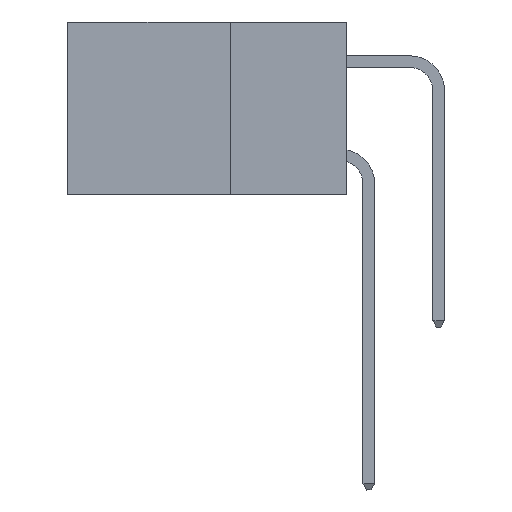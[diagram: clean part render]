
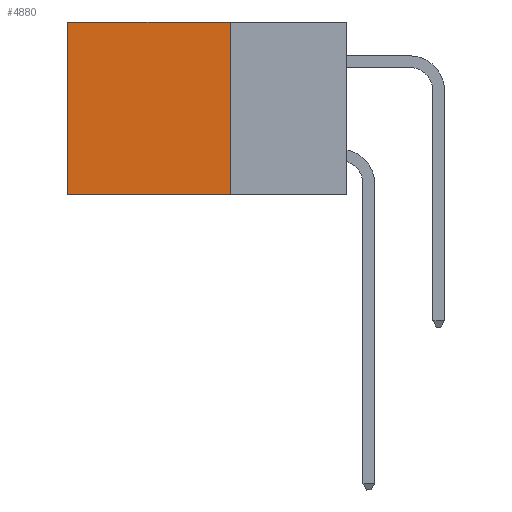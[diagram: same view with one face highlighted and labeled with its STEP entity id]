
A CAD part, left-side view. The second image highlights one B-rep face of the part: STEP entity #4880.
In plain terms, the highlighted planar face has unit normal (-1, 0, 0).
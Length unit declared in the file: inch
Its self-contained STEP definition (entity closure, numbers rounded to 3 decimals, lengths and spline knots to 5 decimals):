
#574 = CARTESIAN_POINT ( 'NONE',  ( 0.2875, 0.25, 0. ) ) ;
#4880 = ADVANCED_FACE ( 'NONE', ( #31165 ), #34774, .F. ) ;
#5216 = EDGE_LOOP ( 'NONE', ( #14999, #32293, #36524, #15111 ) ) ;
#5328 = DIRECTION ( 'NONE',  ( 0., 1., 0. ) ) ;
#6988 = DIRECTION ( 'NONE',  ( 0., 1., 0. ) ) ;
#8904 = VERTEX_POINT ( 'NONE', #18825 ) ;
#9302 = EDGE_CURVE ( 'NONE', #16765, #35006, #14857, .T. ) ;
#9684 = CARTESIAN_POINT ( 'NONE',  ( 0.2875, 0.25, 0. ) ) ;
#10990 = VECTOR ( 'NONE', #6988, 39.37008 ) ;
#11474 = DIRECTION ( 'NONE',  ( 1., 0., 0. ) ) ;
#12344 = EDGE_CURVE ( 'NONE', #27706, #8904, #24925, .T. ) ;
#14065 = LINE ( 'NONE', #31972, #17179 ) ;
#14857 = LINE ( 'NONE', #25021, #18879 ) ;
#14999 = ORIENTED_EDGE ( 'NONE', *, *, #33386, .T. ) ;
#15111 = ORIENTED_EDGE ( 'NONE', *, *, #12344, .T. ) ;
#16765 = VERTEX_POINT ( 'NONE', #18078 ) ;
#17179 = VECTOR ( 'NONE', #25967, 39.37008 ) ;
#18078 = CARTESIAN_POINT ( 'NONE',  ( 0.2875, 0.25, -0.37 ) ) ;
#18412 = CARTESIAN_POINT ( 'NONE',  ( 0.2875, 0.25, 0. ) ) ;
#18825 = CARTESIAN_POINT ( 'NONE',  ( 0.2875, 0.6, 0. ) ) ;
#18879 = VECTOR ( 'NONE', #5328, 39.37008 ) ;
#19658 = CARTESIAN_POINT ( 'NONE',  ( 0.2875, 0.6, -0.37 ) ) ;
#20330 = AXIS2_PLACEMENT_3D ( 'NONE', #574, #11474, #23914 ) ;
#23914 = DIRECTION ( 'NONE',  ( 0., 0., -1. ) ) ;
#24255 = DIRECTION ( 'NONE',  ( 0., 0., -1. ) ) ;
#24925 = LINE ( 'NONE', #18412, #10990 ) ;
#25021 = CARTESIAN_POINT ( 'NONE',  ( 0.2875, 0.25, -0.37 ) ) ;
#25967 = DIRECTION ( 'NONE',  ( 0., 0., -1. ) ) ;
#26576 = VECTOR ( 'NONE', #24255, 39.37008 ) ;
#27706 = VERTEX_POINT ( 'NONE', #27830 ) ;
#27830 = CARTESIAN_POINT ( 'NONE',  ( 0.2875, 0.25, 0. ) ) ;
#31165 = FACE_OUTER_BOUND ( 'NONE', #5216, .T. ) ;
#31972 = CARTESIAN_POINT ( 'NONE',  ( 0.2875, 0.6, 0. ) ) ;
#32293 = ORIENTED_EDGE ( 'NONE', *, *, #9302, .F. ) ;
#32823 = LINE ( 'NONE', #9684, #26576 ) ;
#33386 = EDGE_CURVE ( 'NONE', #8904, #35006, #14065, .T. ) ;
#34060 = EDGE_CURVE ( 'NONE', #27706, #16765, #32823, .T. ) ;
#34774 = PLANE ( 'NONE',  #20330 ) ;
#35006 = VERTEX_POINT ( 'NONE', #19658 ) ;
#36524 = ORIENTED_EDGE ( 'NONE', *, *, #34060, .F. ) ;
